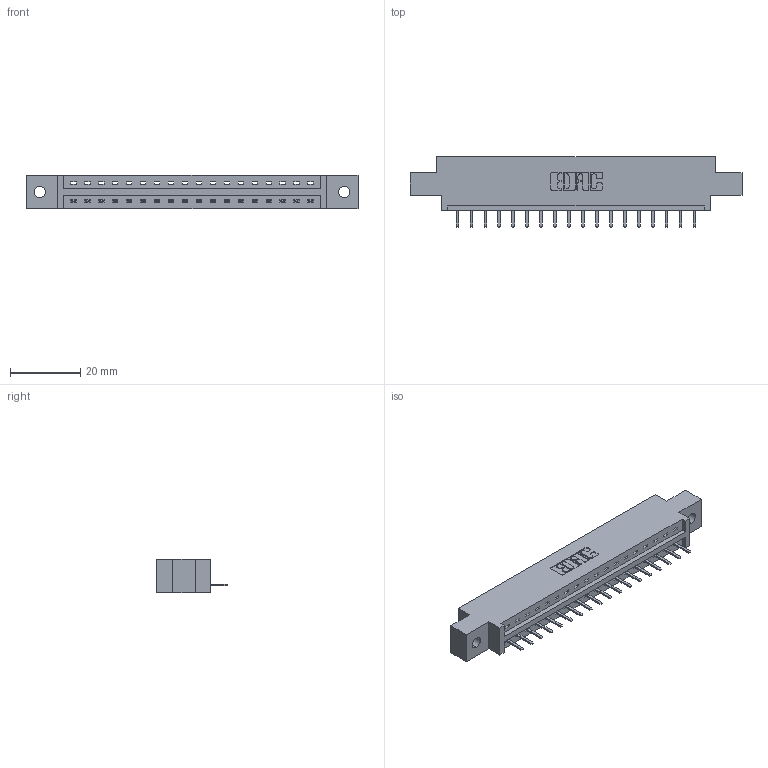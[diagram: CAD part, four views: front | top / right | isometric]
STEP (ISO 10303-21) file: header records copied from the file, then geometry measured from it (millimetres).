
FILE_DESCRIPTION (( 'STEP AP203' ), '1' );
FILE_NAME ('337-018-520-602.STEP', '2018-08-04T23:20:53', ( '' ), ( '' ), 'SwSTEP 2.0', 'SolidWorks 2016', '' );
FILE_SCHEMA (( 'CONFIG_CONTROL_DESIGN' ));
Length unit declared in the file: inch
Products named in the file (3): 337 Part_0.170 Offset - 0.128 Dia; 345-292-001_345-293-120; 337-018-520-602
Assembly tree (19 placements, depth 2):
  337-018-520-602
    337 Part_0.170 Offset - 0.128 Dia
    345-292-001_345-293-120  x18
Bounding box: 94.34 x 20.02 x 9.4 mm (x, y, z)
Volume: 9298.3 mm3; surface area: 9115.4 mm2
Topology: 19 solids, 19 shells, 1306 faces, 3851 edges, 2518 vertices
Faces by surface type: plane 938, cylinder 368
Entity records: 16733 total; most frequent: CARTESIAN_POINT 2932, ORIENTED_EDGE 2874, DIRECTION 2505, EDGE_CURVE 1437, LINE 1305, VECTOR 1305, VERTEX_POINT 954, AXIS2_PLACEMENT_3D 600
